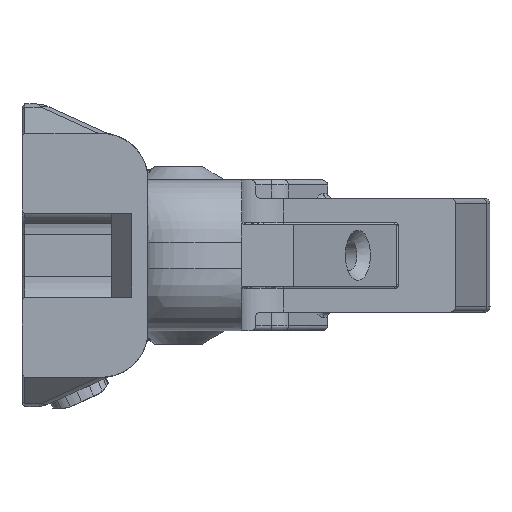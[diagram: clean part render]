
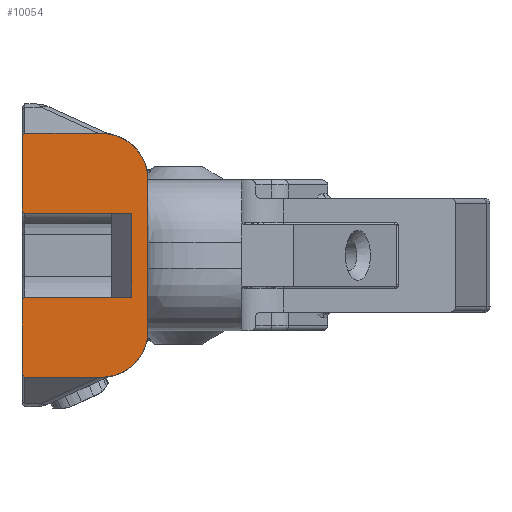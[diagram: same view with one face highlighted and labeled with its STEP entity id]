
A CAD part, left-side view. The second image highlights one B-rep face of the part: STEP entity #10054.
In plain terms, the highlighted planar face has unit normal (-1, 0, 0).
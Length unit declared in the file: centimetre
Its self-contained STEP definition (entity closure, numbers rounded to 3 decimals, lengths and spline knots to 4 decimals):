
#327=PLANE($,#10873);
#1163=FACE_OUTER_BOUND($,#1826,.T.);
#1826=EDGE_LOOP($,(#9280,#9281,#9282,#9283,#9284,#9285,#9286,#9287,#9288,
#9289,#9290,#9291,#9292,#9293));
#2341=CIRCLE($,#10263,0.7057);
#2556=CIRCLE($,#10874,0.7057);
#2593=LINE($,#14639,#3281);
#2627=LINE($,#15005,#3315);
#2638=LINE($,#15134,#3326);
#3218=LINE($,#23885,#3906);
#3220=LINE($,#23889,#3908);
#3222=LINE($,#23893,#3910);
#3224=LINE($,#23897,#3912);
#3226=LINE($,#23900,#3914);
#3227=LINE($,#23902,#3915);
#3229=LINE($,#23906,#3917);
#3231=LINE($,#23910,#3919);
#3233=LINE($,#23913,#3921);
#3281=VECTOR($,#11118,2.3019);
#3315=VECTOR($,#11238,1.172);
#3326=VECTOR($,#11303,1.172);
#3906=VECTOR($,#13103,1.63);
#3908=VECTOR($,#13107,0.0566);
#3910=VECTOR($,#13111,0.0566);
#3912=VECTOR($,#13115,0.0566);
#3914=VECTOR($,#13119,1.1417);
#3915=VECTOR($,#13120,1.1417);
#3917=VECTOR($,#13124,0.0566);
#3919=VECTOR($,#13128,1.63);
#3921=VECTOR($,#13132,1.27);
#4036=VERTEX_POINT($,#14636);
#4037=VERTEX_POINT($,#14638);
#4103=VERTEX_POINT($,#15002);
#4104=VERTEX_POINT($,#15004);
#4131=VERTEX_POINT($,#15131);
#4132=VERTEX_POINT($,#15133);
#4869=VERTEX_POINT($,#23882);
#4870=VERTEX_POINT($,#23884);
#4871=VERTEX_POINT($,#23888);
#4872=VERTEX_POINT($,#23892);
#4873=VERTEX_POINT($,#23896);
#4874=VERTEX_POINT($,#23901);
#4875=VERTEX_POINT($,#23905);
#4876=VERTEX_POINT($,#23909);
#5028=EDGE_CURVE($,#4036,#4037,#2593,.T.);
#5102=EDGE_CURVE($,#4103,#4104,#2627,.F.);
#5133=EDGE_CURVE($,#4131,#4132,#2638,.T.);
#5156=EDGE_CURVE($,#4037,#4131,#2341,.T.);
#6321=EDGE_CURVE($,#4869,#4870,#3218,.F.);
#6323=EDGE_CURVE($,#4870,#4871,#3220,.T.);
#6325=EDGE_CURVE($,#4872,#4103,#3222,.T.);
#6327=EDGE_CURVE($,#4132,#4873,#3224,.T.);
#6329=EDGE_CURVE($,#4871,#4872,#3226,.T.);
#6330=EDGE_CURVE($,#4873,#4874,#3227,.T.);
#6332=EDGE_CURVE($,#4874,#4875,#3229,.T.);
#6334=EDGE_CURVE($,#4875,#4876,#3231,.T.);
#6336=EDGE_CURVE($,#4876,#4869,#3233,.F.);
#6363=EDGE_CURVE($,#4104,#4036,#2556,.T.);
#9280=ORIENTED_EDGE($,*,*,#6336,.F.);
#9281=ORIENTED_EDGE($,*,*,#6334,.F.);
#9282=ORIENTED_EDGE($,*,*,#6332,.F.);
#9283=ORIENTED_EDGE($,*,*,#6330,.F.);
#9284=ORIENTED_EDGE($,*,*,#6327,.F.);
#9285=ORIENTED_EDGE($,*,*,#5133,.F.);
#9286=ORIENTED_EDGE($,*,*,#5156,.F.);
#9287=ORIENTED_EDGE($,*,*,#5028,.F.);
#9288=ORIENTED_EDGE($,*,*,#6363,.F.);
#9289=ORIENTED_EDGE($,*,*,#5102,.F.);
#9290=ORIENTED_EDGE($,*,*,#6325,.F.);
#9291=ORIENTED_EDGE($,*,*,#6329,.F.);
#9292=ORIENTED_EDGE($,*,*,#6323,.F.);
#9293=ORIENTED_EDGE($,*,*,#6321,.F.);
#10054=ADVANCED_FACE($,(#1163),#327,.F.);
#10263=AXIS2_PLACEMENT_3D($,#15513,#11369,#11370);
#10873=AXIS2_PLACEMENT_3D($,#24861,#13190,#13191);
#10874=AXIS2_PLACEMENT_3D($,#24862,#13192,#13193);
#11118=DIRECTION($,(0.,0.,-1.));
#11238=DIRECTION($,(0.,1.,0.));
#11303=DIRECTION($,(0.,1.,0.));
#11369=DIRECTION('center_axis',(1.,0.,0.));
#11370=DIRECTION('ref_axis',(0.,0.,
1.));
#13103=DIRECTION($,(0.,-1.,0.));
#13107=DIRECTION($,(0.,0.707,0.707));
#13111=DIRECTION($,(0.,-0.707,0.707));
#13115=DIRECTION($,(0.,0.707,0.707));
#13119=DIRECTION($,(0.,0.,1.));
#13120=DIRECTION($,(0.,0.,1.));
#13124=DIRECTION($,(0.,-0.707,0.707));
#13128=DIRECTION($,(0.,-1.,0.));
#13132=DIRECTION($,(0.,0.,-1.));
#13190=DIRECTION('center_axis',(1.,0.,0.));
#13191=DIRECTION('ref_axis',(0.,0.,
-1.));
#13192=DIRECTION('center_axis',(1.,0.,0.));
#13193=DIRECTION('ref_axis',(0.,0.,
1.));
#14636=CARTESIAN_POINT('',(-19.5982,-1.3536,1.2509));
#14638=CARTESIAN_POINT('',(-19.5982,-1.3536,-1.0509));
#14639=CARTESIAN_POINT($,(-19.5982,-1.3536,-1.051));
#15002=CARTESIAN_POINT('',(-19.5982,0.5241,1.9567));
#15004=CARTESIAN_POINT('',(-19.5982,-0.6479,1.9567));
#15005=CARTESIAN_POINT($,(-19.5982,-0.2459,1.9567));
#15131=CARTESIAN_POINT('',(-19.5982,-0.6479,-1.7567));
#15133=CARTESIAN_POINT('',(-19.5982,0.5241,-1.7567));
#15134=CARTESIAN_POINT($,(-19.5982,0.1273,-1.7567));
#15513=CARTESIAN_POINT('Origin',(-19.5982,-0.6479,-1.0509));
#23882=CARTESIAN_POINT('',(-19.5982,-1.1059,0.735));
#23884=CARTESIAN_POINT('',(-19.5982,0.5241,0.735));
#23885=CARTESIAN_POINT($,(-19.5982,1.81,0.735));
#23888=CARTESIAN_POINT('',(-19.5982,0.5641,0.775));
#23889=CARTESIAN_POINT($,(-19.5982,-0.1209,0.0901));
#23892=CARTESIAN_POINT('',(-19.5982,0.5641,1.9167));
#23893=CARTESIAN_POINT($,(-19.5982,1.0776,1.4031));
#23896=CARTESIAN_POINT('',(-19.5982,0.5641,-1.7167));
#23897=CARTESIAN_POINT($,(-19.5982,0.5021,-1.7787));
#23900=CARTESIAN_POINT($,(-19.5982,0.5641,-1.6584));
#23901=CARTESIAN_POINT('',(-19.5982,0.5641,-0.575));
#23902=CARTESIAN_POINT($,(-19.5982,0.5641,-1.6584));
#23905=CARTESIAN_POINT('',(-19.5982,0.5241,-0.535));
#23906=CARTESIAN_POINT($,(-19.5982,0.4547,-0.4656));
#23909=CARTESIAN_POINT('',(-19.5982,-1.1059,-0.535));
#23910=CARTESIAN_POINT($,(-19.5982,1.81,-0.535));
#23913=CARTESIAN_POINT($,(-19.5982,-1.1059,-0.4417));
#24861=CARTESIAN_POINT('Origin',(-19.5982,-0.3095,-1.0511));
#24862=CARTESIAN_POINT('Origin',(-19.5982,-0.6479,1.2509));
